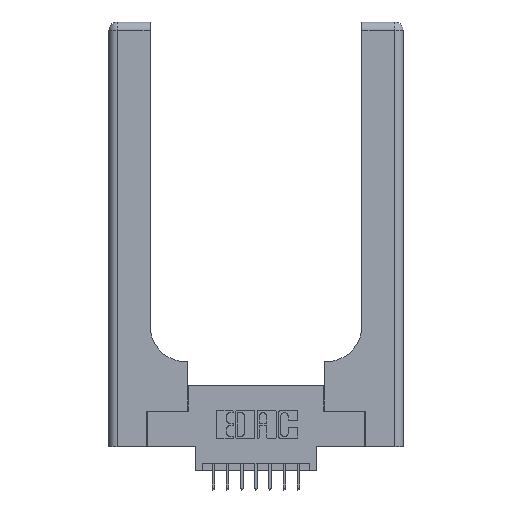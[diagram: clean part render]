
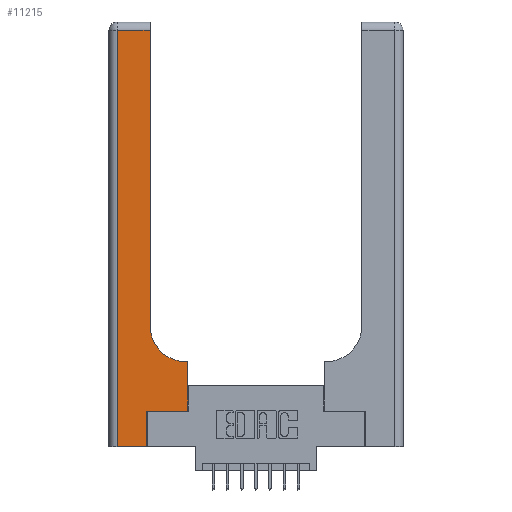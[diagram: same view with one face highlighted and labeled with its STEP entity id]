
A CAD part, top view. The second image highlights one B-rep face of the part: STEP entity #11215.
In plain terms, the highlighted planar face has unit normal (0, 0, 1).
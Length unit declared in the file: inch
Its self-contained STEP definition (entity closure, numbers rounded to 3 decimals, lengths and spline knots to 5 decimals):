
#74 = EDGE_CURVE ( 'NONE', #10060, #13272, #14974, .T. ) ;
#88 = PLANE ( 'NONE',  #14286 ) ;
#365 = DIRECTION ( 'NONE',  ( 1., 0., 0. ) ) ;
#390 = DIRECTION ( 'NONE',  ( 0., 1., 0. ) ) ;
#508 = EDGE_CURVE ( 'NONE', #12454, #1746, #10873, .T. ) ;
#849 = CARTESIAN_POINT ( 'NONE',  ( 0.2915, 0.6, 0.37 ) ) ;
#901 = DIRECTION ( 'NONE',  ( 0., 1., 0. ) ) ;
#1319 = CARTESIAN_POINT ( 'NONE',  ( 0.2915, 0.85, 0.37 ) ) ;
#1373 = CARTESIAN_POINT ( 'NONE',  ( 0.5415, 0.6, 0.37 ) ) ;
#1746 = VERTEX_POINT ( 'NONE', #6170 ) ;
#2067 = DIRECTION ( 'NONE',  ( 0., 1., 0. ) ) ;
#2132 = VECTOR ( 'NONE', #14491, 39.37008 ) ;
#2231 = ORIENTED_EDGE ( 'NONE', *, *, #7936, .T. ) ;
#2496 = CARTESIAN_POINT ( 'NONE',  ( 0.269, 0.25, 0.37 ) ) ;
#3416 = VECTOR ( 'NONE', #901, 39.37008 ) ;
#3489 = DIRECTION ( 'NONE',  ( 0., 0., -1. ) ) ;
#3901 = DIRECTION ( 'NONE',  ( 0., 0., -1. ) ) ;
#4458 = VERTEX_POINT ( 'NONE', #1319 ) ;
#4468 = LINE ( 'NONE', #12708, #3416 ) ;
#4625 = DIRECTION ( 'NONE',  ( 1., 0., 0. ) ) ;
#4817 = CARTESIAN_POINT ( 'NONE',  ( 0., 3., 0.37 ) ) ;
#4829 = AXIS2_PLACEMENT_3D ( 'NONE', #9654, #3489, #11805 ) ;
#5143 = FACE_OUTER_BOUND ( 'NONE', #11837, .T. ) ;
#5278 = ORIENTED_EDGE ( 'NONE', *, *, #10476, .T. ) ;
#5627 = VECTOR ( 'NONE', #6942, 39.37008 ) ;
#5673 = DIRECTION ( 'NONE',  ( -1., 0., 0. ) ) ;
#6170 = CARTESIAN_POINT ( 'NONE',  ( 0.269, 0., 0.37 ) ) ;
#6258 = EDGE_CURVE ( 'NONE', #11386, #12454, #12728, .T. ) ;
#6389 = CARTESIAN_POINT ( 'NONE',  ( 0.5585, 0.25, 0.37 ) ) ;
#6942 = DIRECTION ( 'NONE',  ( 0., -1., 0. ) ) ;
#7318 = ORIENTED_EDGE ( 'NONE', *, *, #74, .T. ) ;
#7366 = VERTEX_POINT ( 'NONE', #2496 ) ;
#7385 = LINE ( 'NONE', #9659, #2132 ) ;
#7630 = CARTESIAN_POINT ( 'NONE',  ( 0.5585, 0.6, 0.37 ) ) ;
#7936 = EDGE_CURVE ( 'NONE', #8979, #11386, #7385, .T. ) ;
#7949 = CARTESIAN_POINT ( 'NONE',  ( 0.06, 2.94, 0.37 ) ) ;
#8161 = CARTESIAN_POINT ( 'NONE',  ( 0.06, 3., 0.37 ) ) ;
#8979 = VERTEX_POINT ( 'NONE', #15466 ) ;
#9235 = VECTOR ( 'NONE', #390, 39.37008 ) ;
#9654 = CARTESIAN_POINT ( 'NONE',  ( 0.5415, 0.85, 0.37 ) ) ;
#9659 = CARTESIAN_POINT ( 'NONE',  ( 0., 2.94, 0.37 ) ) ;
#9677 = CIRCLE ( 'NONE', #4829, 0.25 ) ;
#9720 = VECTOR ( 'NONE', #2067, 39.37008 ) ;
#9832 = EDGE_CURVE ( 'NONE', #4458, #8979, #10606, .T. ) ;
#10060 = VERTEX_POINT ( 'NONE', #7630 ) ;
#10116 = VERTEX_POINT ( 'NONE', #11561 ) ;
#10476 = EDGE_CURVE ( 'NONE', #10116, #10060, #11313, .T. ) ;
#10606 = LINE ( 'NONE', #14326, #9720 ) ;
#10658 = CARTESIAN_POINT ( 'NONE',  ( 0.06, 0., 0.37 ) ) ;
#10873 = LINE ( 'NONE', #13170, #13915 ) ;
#11033 = EDGE_CURVE ( 'NONE', #1746, #7366, #4468, .T. ) ;
#11066 = ORIENTED_EDGE ( 'NONE', *, *, #9832, .T. ) ;
#11210 = CARTESIAN_POINT ( 'NONE',  ( 0.269, 0.25, 0.37 ) ) ;
#11215 = ADVANCED_FACE ( 'NONE', ( #5143 ), #88, .F. ) ;
#11313 = LINE ( 'NONE', #6389, #9235 ) ;
#11348 = VECTOR ( 'NONE', #5673, 39.37008 ) ;
#11386 = VERTEX_POINT ( 'NONE', #7949 ) ;
#11561 = CARTESIAN_POINT ( 'NONE',  ( 0.5585, 0.25, 0.37 ) ) ;
#11805 = DIRECTION ( 'NONE',  ( 1., 0., 0. ) ) ;
#11837 = EDGE_LOOP ( 'NONE', ( #11066, #2231, #13900, #12045, #15198, #14339, #5278, #7318, #15535 ) ) ;
#11996 = VECTOR ( 'NONE', #365, 39.37008 ) ;
#12045 = ORIENTED_EDGE ( 'NONE', *, *, #508, .T. ) ;
#12399 = LINE ( 'NONE', #11210, #11996 ) ;
#12454 = VERTEX_POINT ( 'NONE', #10658 ) ;
#12708 = CARTESIAN_POINT ( 'NONE',  ( 0.269, 0., 0.37 ) ) ;
#12728 = LINE ( 'NONE', #8161, #5627 ) ;
#13060 = EDGE_CURVE ( 'NONE', #7366, #10116, #12399, .T. ) ;
#13170 = CARTESIAN_POINT ( 'NONE',  ( 0., 0., 0.37 ) ) ;
#13272 = VERTEX_POINT ( 'NONE', #1373 ) ;
#13541 = EDGE_CURVE ( 'NONE', #13272, #4458, #9677, .T. ) ;
#13900 = ORIENTED_EDGE ( 'NONE', *, *, #6258, .T. ) ;
#13915 = VECTOR ( 'NONE', #4625, 39.37008 ) ;
#14286 = AXIS2_PLACEMENT_3D ( 'NONE', #4817, #3901, #14567 ) ;
#14326 = CARTESIAN_POINT ( 'NONE',  ( 0.2915, 3., 0.37 ) ) ;
#14339 = ORIENTED_EDGE ( 'NONE', *, *, #13060, .T. ) ;
#14491 = DIRECTION ( 'NONE',  ( -1., 0., 0. ) ) ;
#14567 = DIRECTION ( 'NONE',  ( -1., 0., 0. ) ) ;
#14974 = LINE ( 'NONE', #849, #11348 ) ;
#15198 = ORIENTED_EDGE ( 'NONE', *, *, #11033, .T. ) ;
#15466 = CARTESIAN_POINT ( 'NONE',  ( 0.2915, 2.94, 0.37 ) ) ;
#15535 = ORIENTED_EDGE ( 'NONE', *, *, #13541, .T. ) ;
